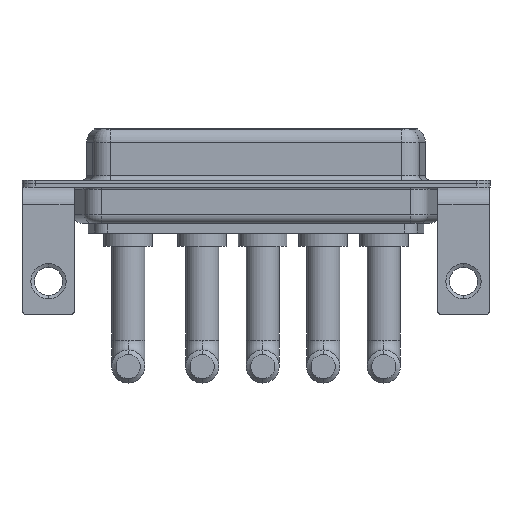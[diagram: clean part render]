
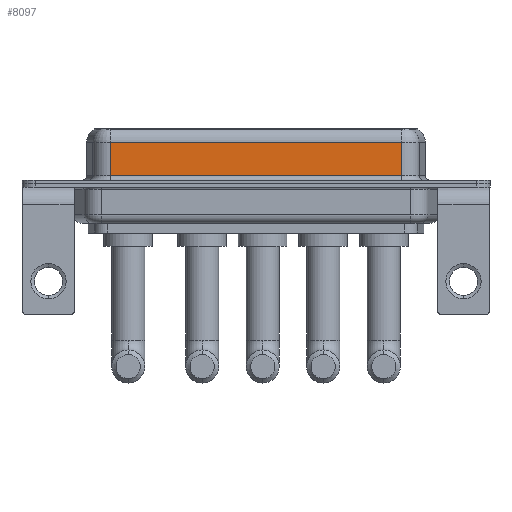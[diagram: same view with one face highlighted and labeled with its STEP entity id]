
A CAD part, front view. The second image highlights one B-rep face of the part: STEP entity #8097.
In plain terms, the highlighted planar face has unit normal (0, -1, 0).
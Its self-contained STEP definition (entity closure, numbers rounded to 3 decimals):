
#95 = VECTOR ( 'NONE', #8727, 1000. ) ;
#385 = LINE ( 'NONE', #508, #11880 ) ;
#508 = CARTESIAN_POINT ( 'NONE',  ( 7.013, -3.95, 6.4 ) ) ;
#593 = DIRECTION ( 'NONE',  ( 0., 0., -1. ) ) ;
#664 = CARTESIAN_POINT ( 'NONE',  ( 40.037, -3.95, 6.4 ) ) ;
#833 = CARTESIAN_POINT ( 'NONE',  ( 7.013, -3.95, 4.65 ) ) ;
#1489 = FACE_OUTER_BOUND ( 'NONE', #4391, .T. ) ;
#1610 = CARTESIAN_POINT ( 'NONE',  ( 40.037, -3.95, 4.65 ) ) ;
#1775 = VERTEX_POINT ( 'NONE', #833 ) ;
#2683 = VERTEX_POINT ( 'NONE', #6170 ) ;
#3128 = ORIENTED_EDGE ( 'NONE', *, *, #9917, .T. ) ;
#3148 = AXIS2_PLACEMENT_3D ( 'NONE', #664, #5662, #9006 ) ;
#3668 = CARTESIAN_POINT ( 'NONE',  ( 40.037, -3.95, 0.9 ) ) ;
#3858 = ORIENTED_EDGE ( 'NONE', *, *, #8593, .T. ) ;
#4227 = VECTOR ( 'NONE', #9957, 1000. ) ;
#4391 = EDGE_LOOP ( 'NONE', ( #4474, #3128, #3858, #10748 ) ) ;
#4474 = ORIENTED_EDGE ( 'NONE', *, *, #12616, .F. ) ;
#4551 = LINE ( 'NONE', #3668, #95 ) ;
#5662 = DIRECTION ( 'NONE',  ( 0., 1., 0. ) ) ;
#5723 = CARTESIAN_POINT ( 'NONE',  ( 40.037, -3.95, 6.4 ) ) ;
#5802 = PLANE ( 'NONE',  #3148 ) ;
#6170 = CARTESIAN_POINT ( 'NONE',  ( 7.013, -3.95, 0.9 ) ) ;
#8097 = ADVANCED_FACE ( 'NONE', ( #1489 ), #5802, .F. ) ;
#8540 = CARTESIAN_POINT ( 'NONE',  ( 40.037, -3.95, 0.9 ) ) ;
#8593 = EDGE_CURVE ( 'NONE', #1775, #2683, #385, .T. ) ;
#8601 = EDGE_CURVE ( 'NONE', #2683, #11961, #4551, .T. ) ;
#8727 = DIRECTION ( 'NONE',  ( 1., 0., 0. ) ) ;
#9006 = DIRECTION ( 'NONE',  ( 0., 0., 1. ) ) ;
#9917 = EDGE_CURVE ( 'NONE', #11830, #1775, #10969, .T. ) ;
#9957 = DIRECTION ( 'NONE',  ( -1., 0., 0. ) ) ;
#10100 = LINE ( 'NONE', #5723, #13313 ) ;
#10748 = ORIENTED_EDGE ( 'NONE', *, *, #8601, .T. ) ;
#10969 = LINE ( 'NONE', #1610, #4227 ) ;
#11051 = DIRECTION ( 'NONE',  ( 0., 0., -1. ) ) ;
#11395 = CARTESIAN_POINT ( 'NONE',  ( 40.037, -3.95, 4.65 ) ) ;
#11830 = VERTEX_POINT ( 'NONE', #11395 ) ;
#11880 = VECTOR ( 'NONE', #11051, 1000. ) ;
#11961 = VERTEX_POINT ( 'NONE', #8540 ) ;
#12616 = EDGE_CURVE ( 'NONE', #11830, #11961, #10100, .T. ) ;
#13313 = VECTOR ( 'NONE', #593, 1000. ) ;
